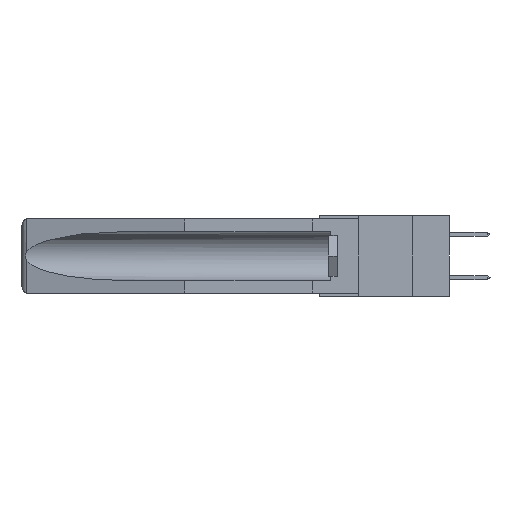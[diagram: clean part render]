
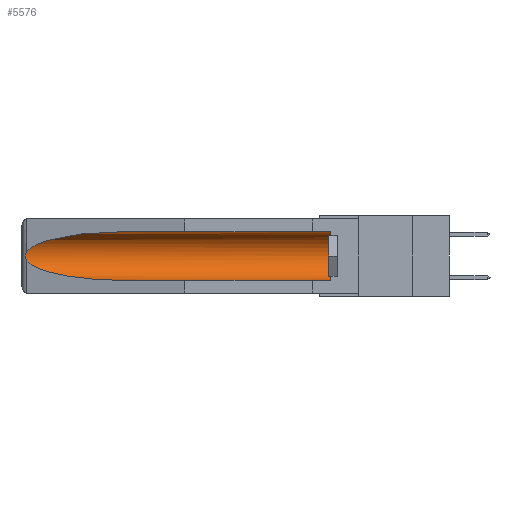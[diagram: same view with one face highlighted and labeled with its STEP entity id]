
A CAD part, left-side view. The second image highlights one B-rep face of the part: STEP entity #5576.
In plain terms, the highlighted cylindrical face has radius 2.857 mm (diameter 5.715 mm), a partial arc.
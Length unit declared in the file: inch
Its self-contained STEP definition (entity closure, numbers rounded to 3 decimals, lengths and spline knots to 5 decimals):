
#614 = CYLINDRICAL_SURFACE ( 'NONE', #1967, 0.1125 ) ;
#796 = CARTESIAN_POINT ( 'NONE',  ( 0.26537, 1.52718, -0.14972 ) ) ;
#834 = CARTESIAN_POINT ( 'NONE',  ( 0.155, -0.30754, -0.059 ) ) ;
#1136 = DIRECTION ( 'NONE',  ( 0., 0., 1. ) ) ;
#1376 = CARTESIAN_POINT ( 'NONE',  ( 0.155, 1.07973, -0.284 ) ) ;
#1715 = CARTESIAN_POINT ( 'NONE',  ( 0.2673, 1.5327, -0.16383 ) ) ;
#1967 = AXIS2_PLACEMENT_3D ( 'NONE', #22624, #18819, #22709 ) ;
#2054 = VERTEX_POINT ( 'NONE', #18748 ) ;
#2223 = CARTESIAN_POINT ( 'NONE',  ( 0.2673, 1.53269, -0.17917 ) ) ;
#3146 = LINE ( 'NONE', #6159, #19443 ) ;
#3747 = ORIENTED_EDGE ( 'NONE', *, *, #21448, .T. ) ;
#4060 = CARTESIAN_POINT ( 'NONE',  ( 0.2675, 1.53308, -0.17534 ) ) ;
#4256 = EDGE_LOOP ( 'NONE', ( #11106, #3747, #14172, #23794, #13972, #13664 ) ) ;
#4806 = B_SPLINE_CURVE_WITH_KNOTS ( 'NONE', 3,
 ( #15027, #9405, #22827, #1715, #11839, #4060, #2223, #17614, #11585, #6100 ),
 .UNSPECIFIED., .F., .F.,
 ( 4, 2, 2, 2, 4 ),
 ( 0., 0.00029, 0.00058, 0.00087, 0.00117 ),
 .UNSPECIFIED. ) ;
#5178 = CARTESIAN_POINT ( 'NONE',  ( 0.25451, 1.48313, -0.24835 ) ) ;
#5426 = CARTESIAN_POINT ( 'NONE',  ( 0.26537, 1.52718, -0.19328 ) ) ;
#5542 = CARTESIAN_POINT ( 'NONE',  ( 0.25451, 1.48313, -0.09465 ) ) ;
#5576 = ADVANCED_FACE ( 'NONE', ( #6047 ), #614, .F. ) ;
#6047 = FACE_OUTER_BOUND ( 'NONE', #4256, .T. ) ;
#6100 = CARTESIAN_POINT ( 'NONE',  ( 0.26537, 1.52718, -0.19328 ) ) ;
#6159 = CARTESIAN_POINT ( 'NONE',  ( 0.155, -0.30754, -0.284 ) ) ;
#6345 =( BOUNDED_CURVE ( )  B_SPLINE_CURVE ( 3, ( #7136, #5178, #14940, #1376 ),
 .UNSPECIFIED., .F., .F. ) 
 B_SPLINE_CURVE_WITH_KNOTS ( ( 4, 4 ),
 ( 0.1948, 1.5708 ),
 .UNSPECIFIED. ) 
 CURVE ( )  GEOMETRIC_REPRESENTATION_ITEM ( )  RATIONAL_B_SPLINE_CURVE ( ( 1., 0.848, 0.848, 1. ) ) 
 REPRESENTATION_ITEM ( '' )  );
#7136 = CARTESIAN_POINT ( 'NONE',  ( 0.26537, 1.52718, -0.19328 ) ) ;
#7322 = CARTESIAN_POINT ( 'NONE',  ( 0.21114, 1.30732, -0.059 ) ) ;
#8267 = DIRECTION ( 'NONE',  ( 0., 1., 0. ) ) ;
#8694 = VERTEX_POINT ( 'NONE', #10337 ) ;
#8695 = DIRECTION ( 'NONE',  ( 0., 1., 0. ) ) ;
#9163 = DIRECTION ( 'NONE',  ( 0., -1., 0. ) ) ;
#9222 = CARTESIAN_POINT ( 'NONE',  ( 0.155, 1.07973, -0.284 ) ) ;
#9405 = CARTESIAN_POINT ( 'NONE',  ( 0.26597, 1.52961, -0.15275 ) ) ;
#10337 = CARTESIAN_POINT ( 'NONE',  ( 0.155, 0.126, -0.284 ) ) ;
#11106 = ORIENTED_EDGE ( 'NONE', *, *, #21909, .T. ) ;
#11585 = CARTESIAN_POINT ( 'NONE',  ( 0.26597, 1.5296, -0.19026 ) ) ;
#11839 = CARTESIAN_POINT ( 'NONE',  ( 0.2675, 1.53308, -0.16763 ) ) ;
#12207 = EDGE_CURVE ( 'NONE', #8694, #2054, #12667, .T. ) ;
#12667 = CIRCLE ( 'NONE', #14804, 0.1125 ) ;
#13664 = ORIENTED_EDGE ( 'NONE', *, *, #19387, .T. ) ;
#13972 = ORIENTED_EDGE ( 'NONE', *, *, #12207, .T. ) ;
#14172 = ORIENTED_EDGE ( 'NONE', *, *, #14222, .T. ) ;
#14222 = EDGE_CURVE ( 'NONE', #20080, #15882, #6345, .T. ) ;
#14804 = AXIS2_PLACEMENT_3D ( 'NONE', #18543, #9163, #1136 ) ;
#14940 = CARTESIAN_POINT ( 'NONE',  ( 0.21114, 1.30732, -0.284 ) ) ;
#15027 = CARTESIAN_POINT ( 'NONE',  ( 0.26537, 1.52718, -0.14972 ) ) ;
#15293 = EDGE_CURVE ( 'NONE', #8694, #15882, #3146, .T. ) ;
#15363 = CARTESIAN_POINT ( 'NONE',  ( 0.155, 1.07973, -0.059 ) ) ;
#15882 = VERTEX_POINT ( 'NONE', #9222 ) ;
#15944 = VECTOR ( 'NONE', #8695, 39.37008 ) ;
#17551 = VERTEX_POINT ( 'NONE', #796 ) ;
#17614 = CARTESIAN_POINT ( 'NONE',  ( 0.26655, 1.53094, -0.18657 ) ) ;
#18543 = CARTESIAN_POINT ( 'NONE',  ( 0.155, 0.126, -0.1715 ) ) ;
#18748 = CARTESIAN_POINT ( 'NONE',  ( 0.155, 0.126, -0.059 ) ) ;
#18819 = DIRECTION ( 'NONE',  ( 0., 1., 0. ) ) ;
#19233 = LINE ( 'NONE', #834, #15944 ) ;
#19387 = EDGE_CURVE ( 'NONE', #2054, #20580, #19233, .T. ) ;
#19443 = VECTOR ( 'NONE', #8267, 39.37008 ) ;
#20080 = VERTEX_POINT ( 'NONE', #5426 ) ;
#20580 = VERTEX_POINT ( 'NONE', #22118 ) ;
#21092 = CARTESIAN_POINT ( 'NONE',  ( 0.26537, 1.52718, -0.14972 ) ) ;
#21448 = EDGE_CURVE ( 'NONE', #17551, #20080, #4806, .T. ) ;
#21909 = EDGE_CURVE ( 'NONE', #20580, #17551, #23139, .T. ) ;
#22118 = CARTESIAN_POINT ( 'NONE',  ( 0.155, 1.07973, -0.059 ) ) ;
#22624 = CARTESIAN_POINT ( 'NONE',  ( 0.155, -0.30754, -0.1715 ) ) ;
#22709 = DIRECTION ( 'NONE',  ( 0., 0., 1. ) ) ;
#22827 = CARTESIAN_POINT ( 'NONE',  ( 0.26654, 1.53092, -0.15636 ) ) ;
#23139 =( BOUNDED_CURVE ( )  B_SPLINE_CURVE ( 3, ( #15363, #7322, #5542, #21092 ),
 .UNSPECIFIED., .F., .F. ) 
 B_SPLINE_CURVE_WITH_KNOTS ( ( 4, 4 ),
 ( 4.71239, 6.08839 ),
 .UNSPECIFIED. ) 
 CURVE ( )  GEOMETRIC_REPRESENTATION_ITEM ( )  RATIONAL_B_SPLINE_CURVE ( ( 1., 0.848, 0.848, 1. ) ) 
 REPRESENTATION_ITEM ( '' )  );
#23794 = ORIENTED_EDGE ( 'NONE', *, *, #15293, .F. ) ;
